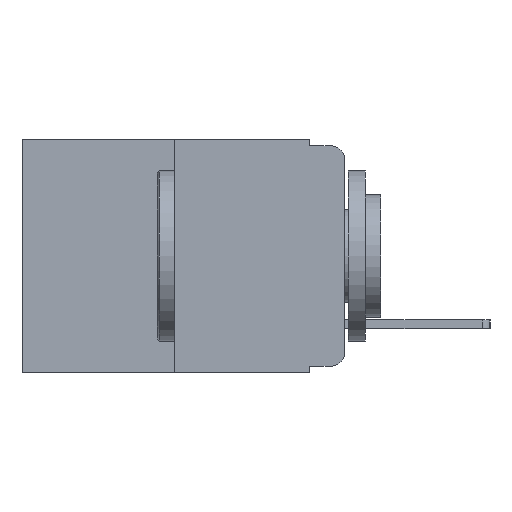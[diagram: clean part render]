
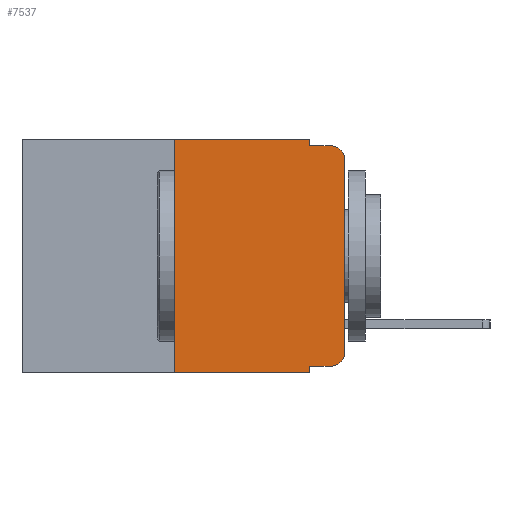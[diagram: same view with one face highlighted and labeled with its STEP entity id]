
A CAD part, left-side view. The second image highlights one B-rep face of the part: STEP entity #7537.
In plain terms, the highlighted planar face has unit normal (-1, 0, 0).
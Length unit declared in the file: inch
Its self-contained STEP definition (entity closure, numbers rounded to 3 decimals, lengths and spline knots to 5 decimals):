
#190 = DIRECTION ( 'NONE',  ( 0., -1., 0. ) ) ;
#194 = EDGE_CURVE ( 'NONE', #4731, #25499, #17562, .T. ) ;
#410 = CARTESIAN_POINT ( 'NONE',  ( 0., 0.02, -0.333 ) ) ;
#505 = EDGE_CURVE ( 'NONE', #16925, #5633, #10810, .T. ) ;
#576 = CARTESIAN_POINT ( 'NONE',  ( 0., 0.051, 0. ) ) ;
#832 = CARTESIAN_POINT ( 'NONE',  ( 0., 0., -0.03 ) ) ;
#918 = CARTESIAN_POINT ( 'NONE',  ( 0., 0.25, 0. ) ) ;
#1000 = CARTESIAN_POINT ( 'NONE',  ( 0., 0.051, -0.333 ) ) ;
#1785 = DIRECTION ( 'NONE',  ( 0., 0., -1. ) ) ;
#1881 = EDGE_LOOP ( 'NONE', ( #25405, #22634, #16072, #12921, #8987, #6750, #20043, #21238, #6141, #10632 ) ) ;
#2078 = VERTEX_POINT ( 'NONE', #8845 ) ;
#2421 = DIRECTION ( 'NONE',  ( 0., 0., 1. ) ) ;
#2970 = LINE ( 'NONE', #23964, #18303 ) ;
#3180 = LINE ( 'NONE', #1000, #18492 ) ;
#3482 = EDGE_CURVE ( 'NONE', #21956, #23928, #19222, .T. ) ;
#3633 = VERTEX_POINT ( 'NONE', #410 ) ;
#3986 = CIRCLE ( 'NONE', #16820, 0.02 ) ;
#4171 = DIRECTION ( 'NONE',  ( -1., 0., 0. ) ) ;
#4731 = VERTEX_POINT ( 'NONE', #17819 ) ;
#4880 = EDGE_CURVE ( 'NONE', #2078, #24989, #2970, .T. ) ;
#4894 = CARTESIAN_POINT ( 'NONE',  ( 0., 0.051, -0.333 ) ) ;
#5182 = CARTESIAN_POINT ( 'NONE',  ( 0., 0.473, 0. ) ) ;
#5633 = VERTEX_POINT ( 'NONE', #22454 ) ;
#5678 = DIRECTION ( 'NONE',  ( 0., 0., -1. ) ) ;
#6141 = ORIENTED_EDGE ( 'NONE', *, *, #6913, .T. ) ;
#6195 = VERTEX_POINT ( 'NONE', #576 ) ;
#6750 = ORIENTED_EDGE ( 'NONE', *, *, #3482, .F. ) ;
#6913 = EDGE_CURVE ( 'NONE', #16925, #3633, #3180, .T. ) ;
#6985 = VECTOR ( 'NONE', #2421, 39.37008 ) ;
#7537 = ADVANCED_FACE ( 'NONE', ( #14875 ), #9706, .F. ) ;
#8215 = LINE ( 'NONE', #10434, #17499 ) ;
#8431 = CIRCLE ( 'NONE', #9316, 0.02 ) ;
#8740 = DIRECTION ( 'NONE',  ( -1., 0., 0. ) ) ;
#8845 = CARTESIAN_POINT ( 'NONE',  ( 0., 0.051, -0.01 ) ) ;
#8951 = EDGE_CURVE ( 'NONE', #3633, #4731, #8431, .T. ) ;
#8987 = ORIENTED_EDGE ( 'NONE', *, *, #14524, .F. ) ;
#9316 = AXIS2_PLACEMENT_3D ( 'NONE', #16248, #4171, #18152 ) ;
#9706 = PLANE ( 'NONE',  #15813 ) ;
#10345 = DIRECTION ( 'NONE',  ( 0., -1., 0. ) ) ;
#10434 = CARTESIAN_POINT ( 'NONE',  ( 0., 0.473, -0.343 ) ) ;
#10632 = ORIENTED_EDGE ( 'NONE', *, *, #8951, .T. ) ;
#10810 = LINE ( 'NONE', #15957, #20516 ) ;
#11003 = CARTESIAN_POINT ( 'NONE',  ( 0., 0.02, -0.01 ) ) ;
#11225 = DIRECTION ( 'NONE',  ( 0., -1., 0. ) ) ;
#11266 = CARTESIAN_POINT ( 'NONE',  ( 0., 0.25, -0.343 ) ) ;
#11339 = DIRECTION ( 'NONE',  ( 0., -1., 0. ) ) ;
#12402 = VECTOR ( 'NONE', #20658, 39.37008 ) ;
#12921 = ORIENTED_EDGE ( 'NONE', *, *, #19311, .F. ) ;
#14524 = EDGE_CURVE ( 'NONE', #23928, #6195, #16258, .T. ) ;
#14875 = FACE_OUTER_BOUND ( 'NONE', #1881, .T. ) ;
#15009 = EDGE_CURVE ( 'NONE', #25499, #24989, #3986, .T. ) ;
#15543 = CARTESIAN_POINT ( 'NONE',  ( 0., 0., 0. ) ) ;
#15720 = CARTESIAN_POINT ( 'NONE',  ( 0., 0.473, 0. ) ) ;
#15813 = AXIS2_PLACEMENT_3D ( 'NONE', #15720, #17638, #5678 ) ;
#15957 = CARTESIAN_POINT ( 'NONE',  ( 0., 0.051, 0. ) ) ;
#16072 = ORIENTED_EDGE ( 'NONE', *, *, #4880, .F. ) ;
#16248 = CARTESIAN_POINT ( 'NONE',  ( 0., 0.02, -0.313 ) ) ;
#16258 = LINE ( 'NONE', #5182, #20716 ) ;
#16820 = AXIS2_PLACEMENT_3D ( 'NONE', #20461, #8740, #22393 ) ;
#16925 = VERTEX_POINT ( 'NONE', #4894 ) ;
#17499 = VECTOR ( 'NONE', #190, 39.37008 ) ;
#17562 = LINE ( 'NONE', #15543, #6985 ) ;
#17638 = DIRECTION ( 'NONE',  ( 1., 0., 0. ) ) ;
#17819 = CARTESIAN_POINT ( 'NONE',  ( 0., 0., -0.313 ) ) ;
#18152 = DIRECTION ( 'NONE',  ( 0., 0., -1. ) ) ;
#18303 = VECTOR ( 'NONE', #10345, 39.37008 ) ;
#18492 = VECTOR ( 'NONE', #11225, 39.37008 ) ;
#18735 = CARTESIAN_POINT ( 'NONE',  ( 0., 0.051, 0. ) ) ;
#19222 = LINE ( 'NONE', #24324, #25004 ) ;
#19311 = EDGE_CURVE ( 'NONE', #6195, #2078, #22648, .T. ) ;
#20043 = ORIENTED_EDGE ( 'NONE', *, *, #23823, .T. ) ;
#20461 = CARTESIAN_POINT ( 'NONE',  ( 0., 0.02, -0.03 ) ) ;
#20516 = VECTOR ( 'NONE', #1785, 39.37008 ) ;
#20658 = DIRECTION ( 'NONE',  ( 0., 0., -1. ) ) ;
#20716 = VECTOR ( 'NONE', #11339, 39.37008 ) ;
#21238 = ORIENTED_EDGE ( 'NONE', *, *, #505, .F. ) ;
#21956 = VERTEX_POINT ( 'NONE', #11266 ) ;
#22393 = DIRECTION ( 'NONE',  ( 0., 0., -1. ) ) ;
#22454 = CARTESIAN_POINT ( 'NONE',  ( 0., 0.051, -0.343 ) ) ;
#22634 = ORIENTED_EDGE ( 'NONE', *, *, #15009, .T. ) ;
#22648 = LINE ( 'NONE', #18735, #12402 ) ;
#23823 = EDGE_CURVE ( 'NONE', #21956, #5633, #8215, .T. ) ;
#23928 = VERTEX_POINT ( 'NONE', #918 ) ;
#23964 = CARTESIAN_POINT ( 'NONE',  ( 0., 0.051, -0.01 ) ) ;
#24324 = CARTESIAN_POINT ( 'NONE',  ( 0., 0.25, 0. ) ) ;
#24989 = VERTEX_POINT ( 'NONE', #11003 ) ;
#25004 = VECTOR ( 'NONE', #25282, 39.37008 ) ;
#25282 = DIRECTION ( 'NONE',  ( 0., 0., 1. ) ) ;
#25405 = ORIENTED_EDGE ( 'NONE', *, *, #194, .T. ) ;
#25499 = VERTEX_POINT ( 'NONE', #832 ) ;
